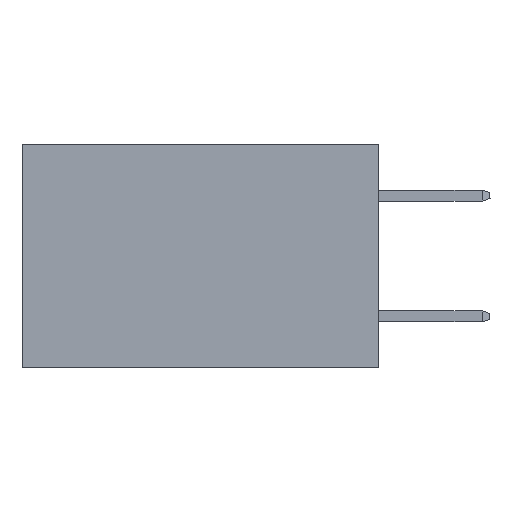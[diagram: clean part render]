
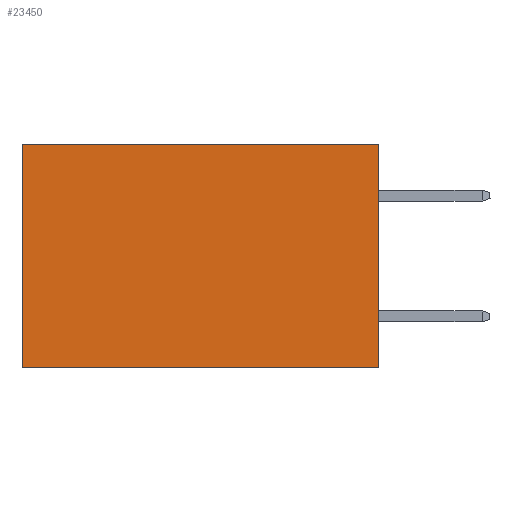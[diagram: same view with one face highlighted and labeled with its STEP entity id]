
A CAD part, left-side view. The second image highlights one B-rep face of the part: STEP entity #23450.
In plain terms, the highlighted planar face has unit normal (-1, 0, 0).
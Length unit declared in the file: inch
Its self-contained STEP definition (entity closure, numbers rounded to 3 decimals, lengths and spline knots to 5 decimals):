
#1086 = VERTEX_POINT ( 'NONE', #24341 ) ;
#1453 = CARTESIAN_POINT ( 'NONE',  ( 0.277, 0.59, -0.37 ) ) ;
#1669 = ORIENTED_EDGE ( 'NONE', *, *, #22778, .T. ) ;
#2093 = CARTESIAN_POINT ( 'NONE',  ( 0.277, 0., -0.37 ) ) ;
#3361 = FACE_OUTER_BOUND ( 'NONE', #6891, .T. ) ;
#3611 = VERTEX_POINT ( 'NONE', #11364 ) ;
#4087 = DIRECTION ( 'NONE',  ( 0., 1., 0. ) ) ;
#4261 = DIRECTION ( 'NONE',  ( 0., 1., 0. ) ) ;
#4372 = VERTEX_POINT ( 'NONE', #18242 ) ;
#6251 = DIRECTION ( 'NONE',  ( 0., 0., -1. ) ) ;
#6891 = EDGE_LOOP ( 'NONE', ( #1669, #18262, #16089, #7673 ) ) ;
#7673 = ORIENTED_EDGE ( 'NONE', *, *, #13672, .T. ) ;
#8574 = CARTESIAN_POINT ( 'NONE',  ( 0.277, 0.59, -0.37 ) ) ;
#8595 = CARTESIAN_POINT ( 'NONE',  ( 0.277, 0., -0.37 ) ) ;
#8966 = VECTOR ( 'NONE', #16289, 39.37008 ) ;
#10562 = DIRECTION ( 'NONE',  ( 1., 0., 0. ) ) ;
#11364 = CARTESIAN_POINT ( 'NONE',  ( 0.277, 0., -0.37 ) ) ;
#12423 = VECTOR ( 'NONE', #4087, 39.37008 ) ;
#13672 = EDGE_CURVE ( 'NONE', #4372, #1086, #24086, .T. ) ;
#15395 = AXIS2_PLACEMENT_3D ( 'NONE', #8595, #10562, #24072 ) ;
#16089 = ORIENTED_EDGE ( 'NONE', *, *, #23922, .F. ) ;
#16289 = DIRECTION ( 'NONE',  ( 0., 0., -1. ) ) ;
#16419 = VERTEX_POINT ( 'NONE', #1453 ) ;
#17593 = LINE ( 'NONE', #2093, #12423 ) ;
#17718 = VECTOR ( 'NONE', #6251, 39.37008 ) ;
#17913 = CARTESIAN_POINT ( 'NONE',  ( 0.277, 0., 0. ) ) ;
#18242 = CARTESIAN_POINT ( 'NONE',  ( 0.277, 0., 0. ) ) ;
#18262 = ORIENTED_EDGE ( 'NONE', *, *, #20612, .F. ) ;
#18930 = LINE ( 'NONE', #19863, #17718 ) ;
#19299 = LINE ( 'NONE', #8574, #8966 ) ;
#19587 = VECTOR ( 'NONE', #4261, 39.37008 ) ;
#19863 = CARTESIAN_POINT ( 'NONE',  ( 0.277, 0., -0.37 ) ) ;
#20218 = PLANE ( 'NONE',  #15395 ) ;
#20612 = EDGE_CURVE ( 'NONE', #3611, #16419, #17593, .T. ) ;
#22778 = EDGE_CURVE ( 'NONE', #1086, #16419, #19299, .T. ) ;
#23450 = ADVANCED_FACE ( 'NONE', ( #3361 ), #20218, .F. ) ;
#23922 = EDGE_CURVE ( 'NONE', #4372, #3611, #18930, .T. ) ;
#24072 = DIRECTION ( 'NONE',  ( 0., 0., -1. ) ) ;
#24086 = LINE ( 'NONE', #17913, #19587 ) ;
#24341 = CARTESIAN_POINT ( 'NONE',  ( 0.277, 0.59, 0. ) ) ;
